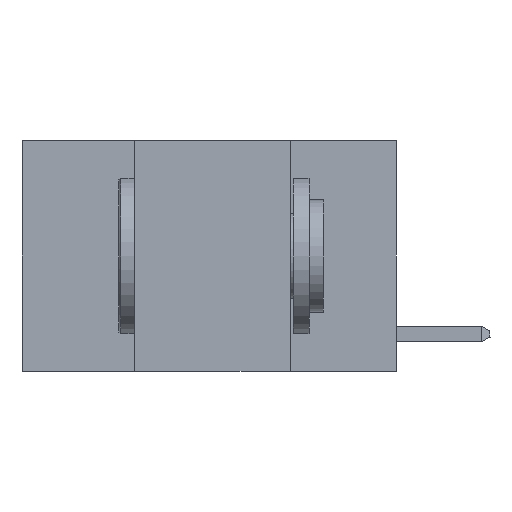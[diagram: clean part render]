
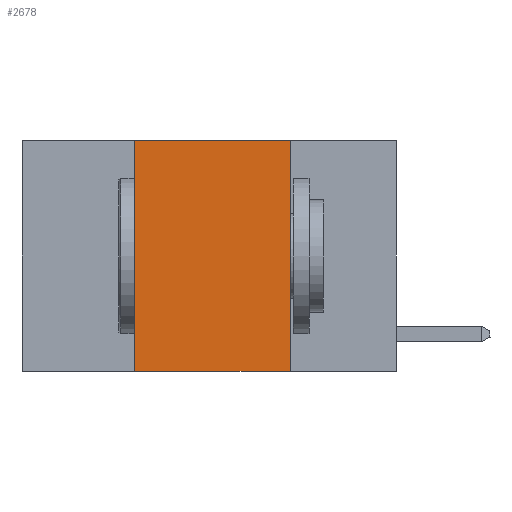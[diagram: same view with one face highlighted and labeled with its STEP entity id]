
A CAD part, left-side view. The second image highlights one B-rep face of the part: STEP entity #2678.
In plain terms, the highlighted planar face has unit normal (-1, 0, 0).
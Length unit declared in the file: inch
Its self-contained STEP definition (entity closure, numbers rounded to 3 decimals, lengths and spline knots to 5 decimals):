
#127 = CARTESIAN_POINT ( 'NONE',  ( 0., 0.42, -0.37 ) ) ;
#640 = EDGE_CURVE ( 'NONE', #22247, #18184, #14590, .T. ) ;
#1493 = CARTESIAN_POINT ( 'NONE',  ( 0., 0.6, 0. ) ) ;
#2302 = CARTESIAN_POINT ( 'NONE',  ( 0., 0.17, -0.37 ) ) ;
#2678 = ADVANCED_FACE ( 'NONE', ( #7141 ), #3174, .F. ) ;
#3174 = PLANE ( 'NONE',  #6543 ) ;
#5286 = DIRECTION ( 'NONE',  ( 0., 0., -1. ) ) ;
#6082 = EDGE_CURVE ( 'NONE', #18184, #23289, #9283, .T. ) ;
#6348 = CARTESIAN_POINT ( 'NONE',  ( 0., 0.17, 0. ) ) ;
#6543 = AXIS2_PLACEMENT_3D ( 'NONE', #9459, #18029, #5286 ) ;
#6644 = VECTOR ( 'NONE', #25468, 39.37008 ) ;
#7141 = FACE_OUTER_BOUND ( 'NONE', #14965, .T. ) ;
#7361 = CARTESIAN_POINT ( 'NONE',  ( 0., 0.6, -0.37 ) ) ;
#9283 = LINE ( 'NONE', #1493, #14978 ) ;
#9459 = CARTESIAN_POINT ( 'NONE',  ( 0., 0.6, 0. ) ) ;
#9492 = EDGE_CURVE ( 'NONE', #23289, #22263, #12269, .T. ) ;
#9736 = DIRECTION ( 'NONE',  ( 0., 0., 1. ) ) ;
#9879 = CARTESIAN_POINT ( 'NONE',  ( 0., 0.17, 0. ) ) ;
#10083 = CARTESIAN_POINT ( 'NONE',  ( 0., 0.42, 0. ) ) ;
#12269 = LINE ( 'NONE', #6348, #6644 ) ;
#13844 = ORIENTED_EDGE ( 'NONE', *, *, #6082, .F. ) ;
#13907 = VECTOR ( 'NONE', #9736, 39.37008 ) ;
#14161 = DIRECTION ( 'NONE',  ( 0., -1., 0. ) ) ;
#14590 = LINE ( 'NONE', #10083, #13907 ) ;
#14965 = EDGE_LOOP ( 'NONE', ( #18170, #13844, #15212, #26431 ) ) ;
#14978 = VECTOR ( 'NONE', #14161, 39.37008 ) ;
#15153 = CARTESIAN_POINT ( 'NONE',  ( 0., 0.42, 0. ) ) ;
#15212 = ORIENTED_EDGE ( 'NONE', *, *, #640, .F. ) ;
#15943 = VECTOR ( 'NONE', #24368, 39.37008 ) ;
#16596 = LINE ( 'NONE', #7361, #15943 ) ;
#18029 = DIRECTION ( 'NONE',  ( 1., 0., 0. ) ) ;
#18170 = ORIENTED_EDGE ( 'NONE', *, *, #9492, .F. ) ;
#18184 = VERTEX_POINT ( 'NONE', #15153 ) ;
#19081 = EDGE_CURVE ( 'NONE', #22247, #22263, #16596, .T. ) ;
#22247 = VERTEX_POINT ( 'NONE', #127 ) ;
#22263 = VERTEX_POINT ( 'NONE', #2302 ) ;
#23289 = VERTEX_POINT ( 'NONE', #9879 ) ;
#24368 = DIRECTION ( 'NONE',  ( 0., -1., 0. ) ) ;
#25468 = DIRECTION ( 'NONE',  ( 0., 0., -1. ) ) ;
#26431 = ORIENTED_EDGE ( 'NONE', *, *, #19081, .T. ) ;
